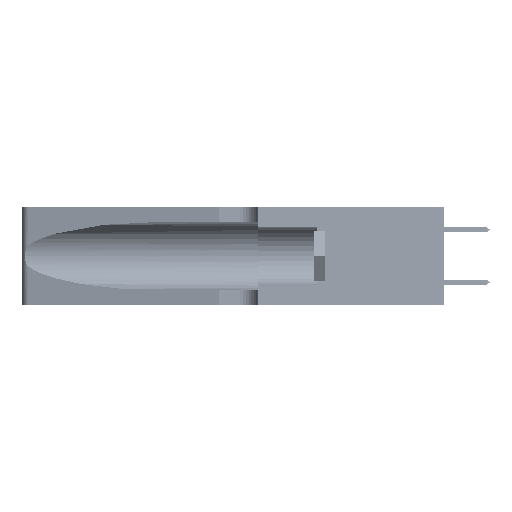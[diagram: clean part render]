
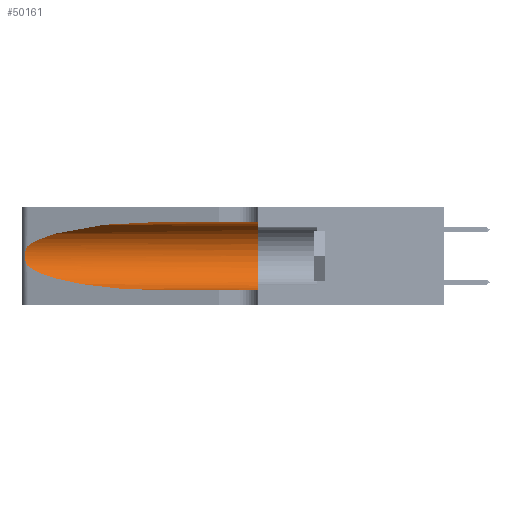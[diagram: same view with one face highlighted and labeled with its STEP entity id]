
A CAD part, left-side view. The second image highlights one B-rep face of the part: STEP entity #50161.
In plain terms, the highlighted cylindrical face has radius 3.308 mm (diameter 6.617 mm), a partial arc.
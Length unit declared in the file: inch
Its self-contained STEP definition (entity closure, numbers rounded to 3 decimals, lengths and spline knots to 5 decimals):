
#213 = CARTESIAN_POINT ( 'NONE',  ( 0.1305, 1.61858, 0.31525 ) ) ;
#871 = CARTESIAN_POINT ( 'NONE',  ( 0.2373, 1.15595, 0.28018 ) ) ;
#1296 = CARTESIAN_POINT ( 'NONE',  ( 0.25487, 1.22718, 0.14631 ) ) ;
#2866 = LINE ( 'NONE', #50736, #43495 ) ;
#3013 = ORIENTED_EDGE ( 'NONE', *, *, #8721, .T. ) ;
#3017 = VERTEX_POINT ( 'NONE', #48967 ) ;
#3078 = CARTESIAN_POINT ( 'NONE',  ( 0.25787, 1.23484, 0.2124 ) ) ;
#4084 = DIRECTION ( 'NONE',  ( 0., 1., 0. ) ) ;
#5615 = EDGE_CURVE ( 'NONE', #36029, #6011, #15378, .T. ) ;
#6001 = CARTESIAN_POINT ( 'NONE',  ( 0.1305, 0.72297, 0.05475 ) ) ;
#6011 = VERTEX_POINT ( 'NONE', #1296 ) ;
#6036 = ORIENTED_EDGE ( 'NONE', *, *, #31998, .F. ) ;
#7071 = CARTESIAN_POINT ( 'NONE',  ( 0.26018, 1.23835, 0.19895 ) ) ;
#7762 = CARTESIAN_POINT ( 'NONE',  ( 0.1305, 0.35, 0.05475 ) ) ;
#7765 =( BOUNDED_CURVE ( )  B_SPLINE_CURVE ( 3, ( #45160, #41266, #29600, #6001 ),
 .UNSPECIFIED., .F., .F. ) 
 B_SPLINE_CURVE_WITH_KNOTS ( ( 4, 4 ),
 ( 3.44316, 4.71239 ),
 .UNSPECIFIED. ) 
 CURVE ( )  GEOMETRIC_REPRESENTATION_ITEM ( )  RATIONAL_B_SPLINE_CURVE ( ( 1., 0.87, 0.87, 1. ) ) 
 REPRESENTATION_ITEM ( '' )  );
#8721 = EDGE_CURVE ( 'NONE', #26136, #39480, #2866, .T. ) ;
#9583 = CYLINDRICAL_SURFACE ( 'NONE', #22628, 0.13025 ) ;
#11068 = CARTESIAN_POINT ( 'NONE',  ( 0.26075, 1.23896, 0.178 ) ) ;
#11624 = DIRECTION ( 'NONE',  ( 0., 0., -1. ) ) ;
#14328 = CARTESIAN_POINT ( 'NONE',  ( 0.25487, 1.22718, 0.22369 ) ) ;
#15032 = CARTESIAN_POINT ( 'NONE',  ( 0.25856, 1.23593, 0.16098 ) ) ;
#15378 = B_SPLINE_CURVE_WITH_KNOTS ( 'NONE', 3,
 ( #26750, #50206, #18817, #3078, #30684, #7071, #34625, #11068, #38590, #15032, #42508, #19003, #46427, #22958 ),
 .UNSPECIFIED., .F., .F.,
 ( 4, 2, 2, 2, 2, 2, 4 ),
 ( 0., 0.00027, 0.00053, 0.00107, 0.0016, 0.00187, 0.00214 ),
 .UNSPECIFIED. ) ;
#16241 = CIRCLE ( 'NONE', #25800, 0.13025 ) ;
#17011 = EDGE_CURVE ( 'NONE', #3017, #17878, #29823, .T. ) ;
#17878 = VERTEX_POINT ( 'NONE', #44237 ) ;
#18817 = CARTESIAN_POINT ( 'NONE',  ( 0.25639, 1.23184, 0.21858 ) ) ;
#19003 = CARTESIAN_POINT ( 'NONE',  ( 0.25639, 1.23186, 0.15144 ) ) ;
#19992 = DIRECTION ( 'NONE',  ( 0., -1., 0. ) ) ;
#20629 = CARTESIAN_POINT ( 'NONE',  ( 0.1305, 0.72297, 0.31525 ) ) ;
#21568 = CARTESIAN_POINT ( 'NONE',  ( 0.1305, 0.72297, 0.05475 ) ) ;
#22628 = AXIS2_PLACEMENT_3D ( 'NONE', #35176, #27287, #11624 ) ;
#22958 = CARTESIAN_POINT ( 'NONE',  ( 0.25487, 1.22718, 0.14631 ) ) ;
#25800 = AXIS2_PLACEMENT_3D ( 'NONE', #27728, #4084, #31664 ) ;
#26136 = VERTEX_POINT ( 'NONE', #21568 ) ;
#26750 = CARTESIAN_POINT ( 'NONE',  ( 0.25487, 1.22718, 0.22369 ) ) ;
#27287 = DIRECTION ( 'NONE',  ( 0., -1., 0. ) ) ;
#27728 = CARTESIAN_POINT ( 'NONE',  ( 0.1305, 0.35, 0.185 ) ) ;
#28525 = CARTESIAN_POINT ( 'NONE',  ( 0.25487, 1.22718, 0.22369 ) ) ;
#29600 = CARTESIAN_POINT ( 'NONE',  ( 0.18966, 0.96281, 0.05475 ) ) ;
#29823 = LINE ( 'NONE', #213, #40242 ) ;
#30531 = FACE_OUTER_BOUND ( 'NONE', #39665, .T. ) ;
#30684 = CARTESIAN_POINT ( 'NONE',  ( 0.25854, 1.2359, 0.20912 ) ) ;
#31664 = DIRECTION ( 'NONE',  ( 0., 0., 1. ) ) ;
#31998 = EDGE_CURVE ( 'NONE', #17878, #39480, #16241, .T. ) ;
#34625 = CARTESIAN_POINT ( 'NONE',  ( 0.26075, 1.23896, 0.19203 ) ) ;
#34941 = EDGE_CURVE ( 'NONE', #3017, #36029, #44299, .T. ) ;
#35176 = CARTESIAN_POINT ( 'NONE',  ( 0.1305, 1.61858, 0.185 ) ) ;
#36029 = VERTEX_POINT ( 'NONE', #14328 ) ;
#38590 = CARTESIAN_POINT ( 'NONE',  ( 0.26017, 1.23833, 0.17102 ) ) ;
#39125 = DIRECTION ( 'NONE',  ( 0., -1., 0. ) ) ;
#39409 = ORIENTED_EDGE ( 'NONE', *, *, #34941, .T. ) ;
#39480 = VERTEX_POINT ( 'NONE', #7762 ) ;
#39665 = EDGE_LOOP ( 'NONE', ( #39409, #41249, #40983, #3013, #6036, #45501 ) ) ;
#40242 = VECTOR ( 'NONE', #19992, 39.37008 ) ;
#40983 = ORIENTED_EDGE ( 'NONE', *, *, #42349, .T. ) ;
#41249 = ORIENTED_EDGE ( 'NONE', *, *, #5615, .T. ) ;
#41266 = CARTESIAN_POINT ( 'NONE',  ( 0.2373, 1.15595, 0.08982 ) ) ;
#42349 = EDGE_CURVE ( 'NONE', #6011, #26136, #7765, .T. ) ;
#42508 = CARTESIAN_POINT ( 'NONE',  ( 0.25789, 1.23486, 0.15765 ) ) ;
#43495 = VECTOR ( 'NONE', #39125, 39.37008 ) ;
#44237 = CARTESIAN_POINT ( 'NONE',  ( 0.1305, 0.35, 0.31525 ) ) ;
#44299 =( BOUNDED_CURVE ( )  B_SPLINE_CURVE ( 3, ( #20629, #48039, #871, #28525 ),
 .UNSPECIFIED., .F., .F. ) 
 B_SPLINE_CURVE_WITH_KNOTS ( ( 4, 4 ),
 ( 1.5708, 2.84003 ),
 .UNSPECIFIED. ) 
 CURVE ( )  GEOMETRIC_REPRESENTATION_ITEM ( )  RATIONAL_B_SPLINE_CURVE ( ( 1., 0.87, 0.87, 1. ) ) 
 REPRESENTATION_ITEM ( '' )  );
#45160 = CARTESIAN_POINT ( 'NONE',  ( 0.25487, 1.22718, 0.14631 ) ) ;
#45501 = ORIENTED_EDGE ( 'NONE', *, *, #17011, .F. ) ;
#46427 = CARTESIAN_POINT ( 'NONE',  ( 0.25555, 1.22993, 0.14849 ) ) ;
#48039 = CARTESIAN_POINT ( 'NONE',  ( 0.18966, 0.96281, 0.31525 ) ) ;
#48967 = CARTESIAN_POINT ( 'NONE',  ( 0.1305, 0.72297, 0.31525 ) ) ;
#50161 = ADVANCED_FACE ( 'NONE', ( #30531 ), #9583, .F. ) ;
#50206 = CARTESIAN_POINT ( 'NONE',  ( 0.25555, 1.22994, 0.2215 ) ) ;
#50736 = CARTESIAN_POINT ( 'NONE',  ( 0.1305, 1.61858, 0.05475 ) ) ;
